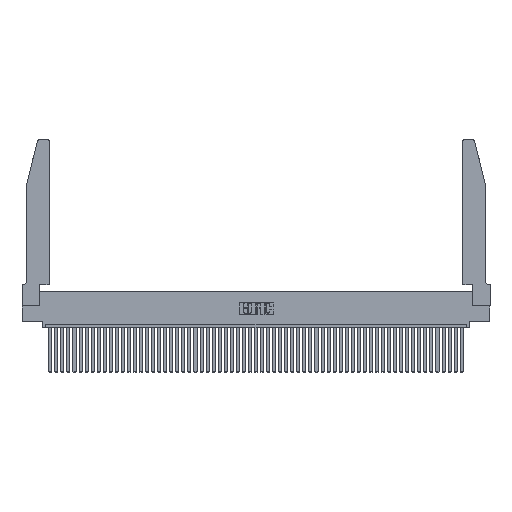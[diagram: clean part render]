
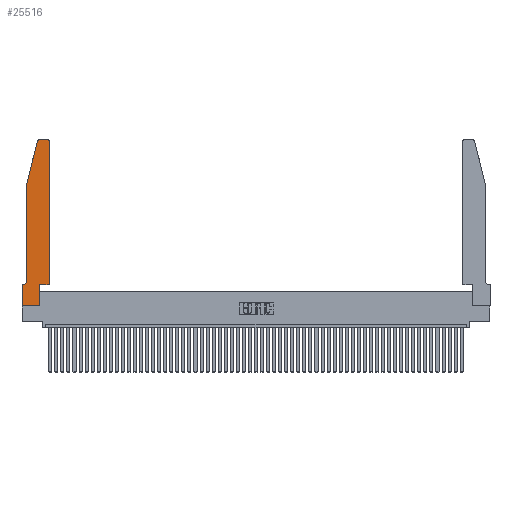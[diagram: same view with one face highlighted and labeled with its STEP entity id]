
A CAD part, top view. The second image highlights one B-rep face of the part: STEP entity #25516.
In plain terms, the highlighted planar face has unit normal (0, 0, 1).
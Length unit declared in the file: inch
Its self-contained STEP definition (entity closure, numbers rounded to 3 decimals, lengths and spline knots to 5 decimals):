
#33 = EDGE_CURVE ( 'NONE', #37718, #32190, #32777, .T. ) ;
#568 = DIRECTION ( 'NONE',  ( 0., -1., 0. ) ) ;
#907 = VERTEX_POINT ( 'NONE', #30098 ) ;
#1674 = CARTESIAN_POINT ( 'NONE',  ( 0.0755, 2., 0.37 ) ) ;
#1943 = DIRECTION ( 'NONE',  ( 1., 0., 0. ) ) ;
#4296 = VERTEX_POINT ( 'NONE', #45935 ) ;
#4784 = VERTEX_POINT ( 'NONE', #40145 ) ;
#4794 = LINE ( 'NONE', #10547, #35676 ) ;
#5177 = ORIENTED_EDGE ( 'NONE', *, *, #33, .T. ) ;
#5366 = EDGE_CURVE ( 'NONE', #25805, #4784, #4794, .T. ) ;
#5412 = CARTESIAN_POINT ( 'NONE',  ( 0.0055, 0.35, 0.37 ) ) ;
#5435 = DIRECTION ( 'NONE',  ( -1., 0., 0. ) ) ;
#5547 = VECTOR ( 'NONE', #35607, 39.37008 ) ;
#5565 = EDGE_LOOP ( 'NONE', ( #51516, #28548, #6456, #15873, #17183, #35527, #5177, #17069, #52260, #52513, #41408, #26288 ) ) ;
#6048 = VERTEX_POINT ( 'NONE', #1674 ) ;
#6340 = CARTESIAN_POINT ( 'NONE',  ( 0.4205, 2.72, 0.37 ) ) ;
#6456 = ORIENTED_EDGE ( 'NONE', *, *, #25705, .T. ) ;
#8566 = EDGE_CURVE ( 'NONE', #4296, #27390, #22516, .T. ) ;
#8848 = EDGE_CURVE ( 'NONE', #6048, #38804, #9658, .T. ) ;
#9032 = VECTOR ( 'NONE', #1943, 39.37008 ) ;
#9266 = DIRECTION ( 'NONE',  ( 1., 0., 0. ) ) ;
#9490 = CARTESIAN_POINT ( 'NONE',  ( 0.0755, 2., 0.37 ) ) ;
#9658 = LINE ( 'NONE', #46164, #39806 ) ;
#9779 = CARTESIAN_POINT ( 'NONE',  ( 0.0055, 0.42, 0.37 ) ) ;
#10107 = DIRECTION ( 'NONE',  ( 0., 0., 1. ) ) ;
#10264 = CARTESIAN_POINT ( 'NONE',  ( 0., 0., 0.37 ) ) ;
#10547 = CARTESIAN_POINT ( 'NONE',  ( 0.2605, 2.75, 0.37 ) ) ;
#13600 = DIRECTION ( 'NONE',  ( -0.239, -0.971, 0. ) ) ;
#13721 = EDGE_CURVE ( 'NONE', #907, #25805, #28508, .T. ) ;
#13738 = CARTESIAN_POINT ( 'NONE',  ( 0.284, 2.72, 0.37 ) ) ;
#14465 = LINE ( 'NONE', #19810, #38762 ) ;
#14950 = CARTESIAN_POINT ( 'NONE',  ( 0., 0.35, 0.37 ) ) ;
#15314 = FACE_OUTER_BOUND ( 'NONE', #5565, .T. ) ;
#15538 = AXIS2_PLACEMENT_3D ( 'NONE', #13738, #21276, #9266 ) ;
#15562 = CARTESIAN_POINT ( 'NONE',  ( 0.2865, 0.35, 0.37 ) ) ;
#15641 = PLANE ( 'NONE',  #32735 ) ;
#15873 = ORIENTED_EDGE ( 'NONE', *, *, #8848, .T. ) ;
#16705 = VERTEX_POINT ( 'NONE', #5412 ) ;
#17069 = ORIENTED_EDGE ( 'NONE', *, *, #29865, .T. ) ;
#17183 = ORIENTED_EDGE ( 'NONE', *, *, #49139, .T. ) ;
#17425 = VERTEX_POINT ( 'NONE', #41891 ) ;
#17924 = CARTESIAN_POINT ( 'NONE',  ( 0.0755, 0.35, 0.37 ) ) ;
#18137 = DIRECTION ( 'NONE',  ( 0., -1., 0. ) ) ;
#19644 = DIRECTION ( 'NONE',  ( 0., 1., 0. ) ) ;
#19810 = CARTESIAN_POINT ( 'NONE',  ( 0.4505, 0.35, 0.37 ) ) ;
#21276 = DIRECTION ( 'NONE',  ( 0., 0., 1. ) ) ;
#22516 = LINE ( 'NONE', #42596, #9032 ) ;
#24272 = AXIS2_PLACEMENT_3D ( 'NONE', #9779, #26073, #5435 ) ;
#25061 = EDGE_CURVE ( 'NONE', #17425, #4296, #39576, .T. ) ;
#25247 = CARTESIAN_POINT ( 'NONE',  ( 0., 0., 0.37 ) ) ;
#25516 = ADVANCED_FACE ( 'NONE', ( #15314 ), #15641, .T. ) ;
#25705 = EDGE_CURVE ( 'NONE', #35409, #6048, #38190, .T. ) ;
#25805 = VERTEX_POINT ( 'NONE', #26386 ) ;
#26073 = DIRECTION ( 'NONE',  ( 0., 0., -1. ) ) ;
#26288 = ORIENTED_EDGE ( 'NONE', *, *, #13721, .T. ) ;
#26386 = CARTESIAN_POINT ( 'NONE',  ( 0.4205, 2.75, 0.37 ) ) ;
#27140 = CARTESIAN_POINT ( 'NONE',  ( 0.0755, 0.42, 0.37 ) ) ;
#27390 = VERTEX_POINT ( 'NONE', #43757 ) ;
#28033 = CARTESIAN_POINT ( 'NONE',  ( 0., 0., 0.37 ) ) ;
#28508 = CIRCLE ( 'NONE', #42206, 0.03 ) ;
#28548 = ORIENTED_EDGE ( 'NONE', *, *, #33456, .T. ) ;
#28926 = CIRCLE ( 'NONE', #15538, 0.03 ) ;
#29368 = CIRCLE ( 'NONE', #24272, 0.07 ) ;
#29865 = EDGE_CURVE ( 'NONE', #32190, #17425, #37599, .T. ) ;
#30098 = CARTESIAN_POINT ( 'NONE',  ( 0.4505, 2.72, 0.37 ) ) ;
#31116 = EDGE_CURVE ( 'NONE', #27390, #907, #14465, .T. ) ;
#32190 = VERTEX_POINT ( 'NONE', #10264 ) ;
#32735 = AXIS2_PLACEMENT_3D ( 'NONE', #44421, #52067, #36730 ) ;
#32777 = LINE ( 'NONE', #25247, #33989 ) ;
#33456 = EDGE_CURVE ( 'NONE', #4784, #35409, #28926, .T. ) ;
#33771 = EDGE_CURVE ( 'NONE', #16705, #37718, #41617, .T. ) ;
#33989 = VECTOR ( 'NONE', #568, 39.37008 ) ;
#34622 = DIRECTION ( 'NONE',  ( 1., 0., 0. ) ) ;
#35409 = VERTEX_POINT ( 'NONE', #46889 ) ;
#35527 = ORIENTED_EDGE ( 'NONE', *, *, #33771, .T. ) ;
#35607 = DIRECTION ( 'NONE',  ( 0., 1., 0. ) ) ;
#35676 = VECTOR ( 'NONE', #43470, 39.37008 ) ;
#36730 = DIRECTION ( 'NONE',  ( 1., 0., 0. ) ) ;
#37599 = LINE ( 'NONE', #28033, #42052 ) ;
#37718 = VERTEX_POINT ( 'NONE', #14950 ) ;
#38190 = LINE ( 'NONE', #9490, #38889 ) ;
#38762 = VECTOR ( 'NONE', #19644, 39.37008 ) ;
#38804 = VERTEX_POINT ( 'NONE', #27140 ) ;
#38889 = VECTOR ( 'NONE', #13600, 39.37008 ) ;
#39576 = LINE ( 'NONE', #15562, #5547 ) ;
#39806 = VECTOR ( 'NONE', #18137, 39.37008 ) ;
#40145 = CARTESIAN_POINT ( 'NONE',  ( 0.284, 2.75, 0.37 ) ) ;
#40408 = VECTOR ( 'NONE', #46467, 39.37008 ) ;
#41408 = ORIENTED_EDGE ( 'NONE', *, *, #31116, .T. ) ;
#41617 = LINE ( 'NONE', #17924, #40408 ) ;
#41891 = CARTESIAN_POINT ( 'NONE',  ( 0.2865, 0., 0.37 ) ) ;
#42052 = VECTOR ( 'NONE', #44449, 39.37008 ) ;
#42206 = AXIS2_PLACEMENT_3D ( 'NONE', #6340, #10107, #34622 ) ;
#42596 = CARTESIAN_POINT ( 'NONE',  ( 0.4505, 0.35, 0.37 ) ) ;
#43470 = DIRECTION ( 'NONE',  ( -1., 0., 0. ) ) ;
#43757 = CARTESIAN_POINT ( 'NONE',  ( 0.4505, 0.35, 0.37 ) ) ;
#44421 = CARTESIAN_POINT ( 'NONE',  ( 0., 0.35, 0.37 ) ) ;
#44449 = DIRECTION ( 'NONE',  ( 1., 0., 0. ) ) ;
#45935 = CARTESIAN_POINT ( 'NONE',  ( 0.2865, 0.35, 0.37 ) ) ;
#46164 = CARTESIAN_POINT ( 'NONE',  ( 0.0755, 2., 0.37 ) ) ;
#46467 = DIRECTION ( 'NONE',  ( -1., 0., 0. ) ) ;
#46889 = CARTESIAN_POINT ( 'NONE',  ( 0.25487, 2.72718, 0.37 ) ) ;
#49139 = EDGE_CURVE ( 'NONE', #38804, #16705, #29368, .T. ) ;
#51516 = ORIENTED_EDGE ( 'NONE', *, *, #5366, .T. ) ;
#52067 = DIRECTION ( 'NONE',  ( 0., 0., 1. ) ) ;
#52260 = ORIENTED_EDGE ( 'NONE', *, *, #25061, .T. ) ;
#52513 = ORIENTED_EDGE ( 'NONE', *, *, #8566, .T. ) ;
